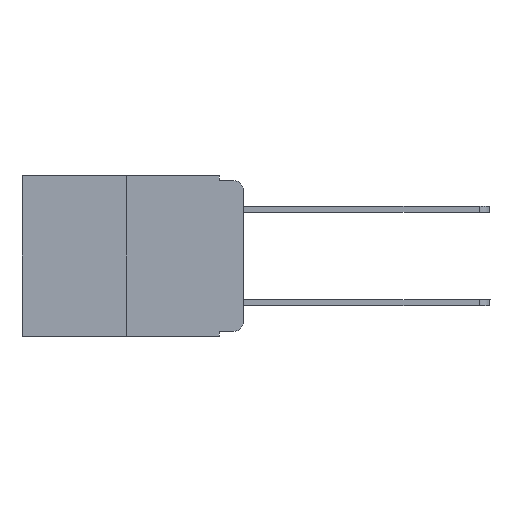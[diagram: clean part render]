
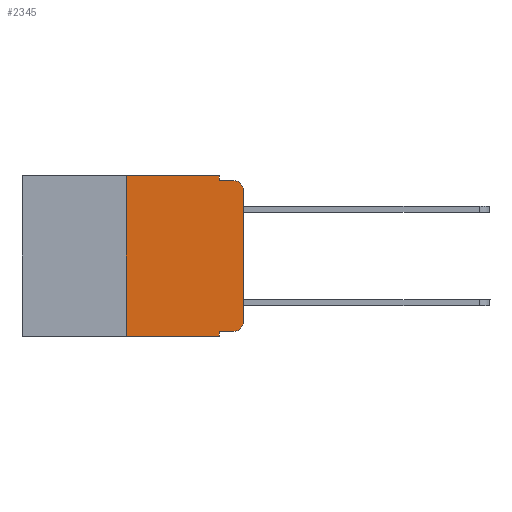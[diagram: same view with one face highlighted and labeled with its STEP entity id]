
A CAD part, left-side view. The second image highlights one B-rep face of the part: STEP entity #2345.
In plain terms, the highlighted planar face has unit normal (-1, 0, 0).
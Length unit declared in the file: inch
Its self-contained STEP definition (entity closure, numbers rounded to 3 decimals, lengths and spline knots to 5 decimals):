
#410 = CIRCLE ( 'NONE', #9328, 0.02 ) ;
#494 = CARTESIAN_POINT ( 'NONE',  ( 0., 0., 0. ) ) ;
#522 = VERTEX_POINT ( 'NONE', #5493 ) ;
#531 = CARTESIAN_POINT ( 'NONE',  ( 0., 0.25, 0. ) ) ;
#655 = DIRECTION ( 'NONE',  ( 0., -1., 0. ) ) ;
#675 = ORIENTED_EDGE ( 'NONE', *, *, #729, .F. ) ;
#729 = EDGE_CURVE ( 'NONE', #2742, #7209, #808, .T. ) ;
#808 = LINE ( 'NONE', #9677, #6408 ) ;
#968 = EDGE_CURVE ( 'NONE', #11686, #11738, #11195, .T. ) ;
#1275 = EDGE_CURVE ( 'NONE', #7209, #522, #13100, .T. ) ;
#1478 = VERTEX_POINT ( 'NONE', #6925 ) ;
#1605 = EDGE_CURVE ( 'NONE', #10098, #522, #11978, .T. ) ;
#1644 = CARTESIAN_POINT ( 'NONE',  ( 0., 0., -0.313 ) ) ;
#1687 = ORIENTED_EDGE ( 'NONE', *, *, #9307, .T. ) ;
#1790 = VERTEX_POINT ( 'NONE', #7885 ) ;
#1898 = VECTOR ( 'NONE', #8333, 39.37008 ) ;
#2311 = DIRECTION ( 'NONE',  ( 0., 0., 1. ) ) ;
#2345 = ADVANCED_FACE ( 'NONE', ( #6372 ), #9699, .F. ) ;
#2582 = DIRECTION ( 'NONE',  ( 1., 0., 0. ) ) ;
#2742 = VERTEX_POINT ( 'NONE', #7786 ) ;
#3390 = ORIENTED_EDGE ( 'NONE', *, *, #8823, .F. ) ;
#3863 = ORIENTED_EDGE ( 'NONE', *, *, #968, .F. ) ;
#3884 = DIRECTION ( 'NONE',  ( -1., 0., 0. ) ) ;
#3980 = ORIENTED_EDGE ( 'NONE', *, *, #9555, .T. ) ;
#4367 = DIRECTION ( 'NONE',  ( 0., -1., 0. ) ) ;
#4547 = CARTESIAN_POINT ( 'NONE',  ( 0., 0.473, 0. ) ) ;
#4559 = VECTOR ( 'NONE', #11844, 39.37008 ) ;
#4563 = DIRECTION ( 'NONE',  ( -1., 0., 0. ) ) ;
#4586 = LINE ( 'NONE', #8703, #1898 ) ;
#4587 = VECTOR ( 'NONE', #655, 39.37008 ) ;
#4765 = VECTOR ( 'NONE', #9195, 39.37008 ) ;
#4893 = EDGE_LOOP ( 'NONE', ( #1687, #12917, #12667, #675, #3390, #12992, #6985, #3863, #4946, #3980 ) ) ;
#4946 = ORIENTED_EDGE ( 'NONE', *, *, #5565, .T. ) ;
#5493 = CARTESIAN_POINT ( 'NONE',  ( 0., 0.02, -0.01 ) ) ;
#5565 = EDGE_CURVE ( 'NONE', #11686, #1790, #10291, .T. ) ;
#5670 = DIRECTION ( 'NONE',  ( 0., 0., -1. ) ) ;
#6279 = CARTESIAN_POINT ( 'NONE',  ( 0., 0., -0.03 ) ) ;
#6372 = FACE_OUTER_BOUND ( 'NONE', #4893, .T. ) ;
#6408 = VECTOR ( 'NONE', #5670, 39.37008 ) ;
#6588 = CARTESIAN_POINT ( 'NONE',  ( 0., 0.02, -0.03 ) ) ;
#6619 = CARTESIAN_POINT ( 'NONE',  ( 0., 0.051, -0.01 ) ) ;
#6850 = CARTESIAN_POINT ( 'NONE',  ( 0., 0.473, 0. ) ) ;
#6925 = CARTESIAN_POINT ( 'NONE',  ( 0., 0.25, -0.343 ) ) ;
#6985 = ORIENTED_EDGE ( 'NONE', *, *, #12442, .T. ) ;
#7209 = VERTEX_POINT ( 'NONE', #11888 ) ;
#7276 = CARTESIAN_POINT ( 'NONE',  ( 0., 0.051, -0.333 ) ) ;
#7318 = CARTESIAN_POINT ( 'NONE',  ( 0., 0.051, -0.343 ) ) ;
#7556 = DIRECTION ( 'NONE',  ( 0., 0., -1. ) ) ;
#7576 = VECTOR ( 'NONE', #9500, 39.37008 ) ;
#7786 = CARTESIAN_POINT ( 'NONE',  ( 0., 0.051, 0. ) ) ;
#7885 = CARTESIAN_POINT ( 'NONE',  ( 0., 0.02, -0.333 ) ) ;
#8061 = VERTEX_POINT ( 'NONE', #531 ) ;
#8259 = LINE ( 'NONE', #494, #4559 ) ;
#8333 = DIRECTION ( 'NONE',  ( 0., -1., 0. ) ) ;
#8703 = CARTESIAN_POINT ( 'NONE',  ( 0., 0.473, -0.343 ) ) ;
#8823 = EDGE_CURVE ( 'NONE', #8061, #2742, #11943, .T. ) ;
#9195 = DIRECTION ( 'NONE',  ( 0., 0., -1. ) ) ;
#9238 = CARTESIAN_POINT ( 'NONE',  ( 0., 0.051, 0. ) ) ;
#9307 = EDGE_CURVE ( 'NONE', #12054, #10098, #8259, .T. ) ;
#9328 = AXIS2_PLACEMENT_3D ( 'NONE', #10010, #3884, #13077 ) ;
#9500 = DIRECTION ( 'NONE',  ( 0., -1., 0. ) ) ;
#9555 = EDGE_CURVE ( 'NONE', #1790, #12054, #410, .T. ) ;
#9677 = CARTESIAN_POINT ( 'NONE',  ( 0., 0.051, 0. ) ) ;
#9699 = PLANE ( 'NONE',  #11743 ) ;
#10010 = CARTESIAN_POINT ( 'NONE',  ( 0., 0.02, -0.313 ) ) ;
#10098 = VERTEX_POINT ( 'NONE', #6279 ) ;
#10291 = LINE ( 'NONE', #11276, #7576 ) ;
#10398 = VECTOR ( 'NONE', #4367, 39.37008 ) ;
#10441 = CARTESIAN_POINT ( 'NONE',  ( 0., 0.25, 0. ) ) ;
#10518 = DIRECTION ( 'NONE',  ( 0., 0., -1. ) ) ;
#11195 = LINE ( 'NONE', #9238, #4765 ) ;
#11276 = CARTESIAN_POINT ( 'NONE',  ( 0., 0.051, -0.333 ) ) ;
#11686 = VERTEX_POINT ( 'NONE', #7276 ) ;
#11738 = VERTEX_POINT ( 'NONE', #7318 ) ;
#11743 = AXIS2_PLACEMENT_3D ( 'NONE', #4547, #2582, #7556 ) ;
#11786 = EDGE_CURVE ( 'NONE', #1478, #8061, #13244, .T. ) ;
#11844 = DIRECTION ( 'NONE',  ( 0., 0., 1. ) ) ;
#11888 = CARTESIAN_POINT ( 'NONE',  ( 0., 0.051, -0.01 ) ) ;
#11943 = LINE ( 'NONE', #6850, #4587 ) ;
#11978 = CIRCLE ( 'NONE', #12930, 0.02 ) ;
#12054 = VERTEX_POINT ( 'NONE', #1644 ) ;
#12276 = VECTOR ( 'NONE', #2311, 39.37008 ) ;
#12442 = EDGE_CURVE ( 'NONE', #1478, #11738, #4586, .T. ) ;
#12667 = ORIENTED_EDGE ( 'NONE', *, *, #1275, .F. ) ;
#12917 = ORIENTED_EDGE ( 'NONE', *, *, #1605, .T. ) ;
#12930 = AXIS2_PLACEMENT_3D ( 'NONE', #6588, #4563, #10518 ) ;
#12992 = ORIENTED_EDGE ( 'NONE', *, *, #11786, .F. ) ;
#13077 = DIRECTION ( 'NONE',  ( 0., 0., -1. ) ) ;
#13100 = LINE ( 'NONE', #6619, #10398 ) ;
#13244 = LINE ( 'NONE', #10441, #12276 ) ;
